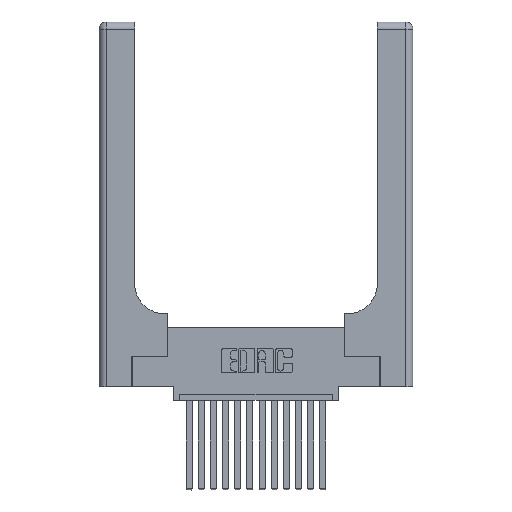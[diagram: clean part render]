
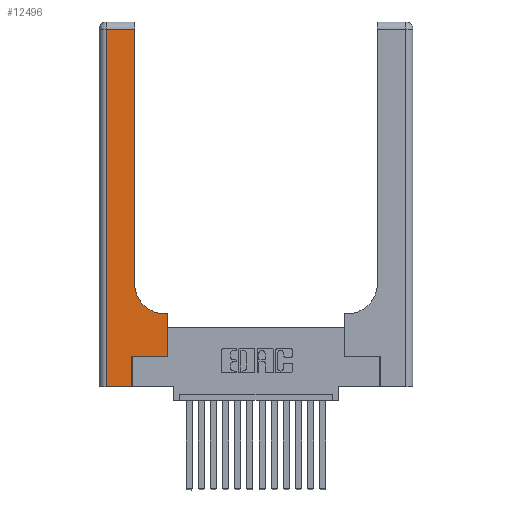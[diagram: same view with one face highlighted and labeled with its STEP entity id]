
A CAD part, top view. The second image highlights one B-rep face of the part: STEP entity #12496.
In plain terms, the highlighted planar face has unit normal (0, 0, 1).
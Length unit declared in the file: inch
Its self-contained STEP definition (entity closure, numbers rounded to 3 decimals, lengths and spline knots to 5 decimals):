
#476 = EDGE_CURVE ( 'NONE', #5047, #6004, #5724, .T. ) ;
#490 = CARTESIAN_POINT ( 'NONE',  ( 0.269, 0., 0.37 ) ) ;
#1063 = ORIENTED_EDGE ( 'NONE', *, *, #13172, .T. ) ;
#1244 = DIRECTION ( 'NONE',  ( 0., 1., 0. ) ) ;
#1622 = DIRECTION ( 'NONE',  ( -1., 0., 0. ) ) ;
#2347 = CARTESIAN_POINT ( 'NONE',  ( 0.269, 0.25, 0.37 ) ) ;
#2625 = EDGE_CURVE ( 'NONE', #14415, #11265, #12244, .T. ) ;
#2713 = CARTESIAN_POINT ( 'NONE',  ( 0.5585, 0.25, 0.37 ) ) ;
#2748 = DIRECTION ( 'NONE',  ( 1., 0., 0. ) ) ;
#2900 = ORIENTED_EDGE ( 'NONE', *, *, #7976, .T. ) ;
#3698 = DIRECTION ( 'NONE',  ( 0., 0., -1. ) ) ;
#3905 = VERTEX_POINT ( 'NONE', #13293 ) ;
#4234 = CARTESIAN_POINT ( 'NONE',  ( 0.2915, 0.6, 0.37 ) ) ;
#4484 = DIRECTION ( 'NONE',  ( 1., 0., 0. ) ) ;
#5047 = VERTEX_POINT ( 'NONE', #8200 ) ;
#5060 = LINE ( 'NONE', #4234, #17176 ) ;
#5097 = DIRECTION ( 'NONE',  ( 1., 0., 0. ) ) ;
#5101 = ORIENTED_EDGE ( 'NONE', *, *, #476, .T. ) ;
#5525 = CARTESIAN_POINT ( 'NONE',  ( 0.06, 3., 0.37 ) ) ;
#5642 = FACE_OUTER_BOUND ( 'NONE', #10318, .T. ) ;
#5724 = LINE ( 'NONE', #11470, #12752 ) ;
#6004 = VERTEX_POINT ( 'NONE', #490 ) ;
#6273 = EDGE_CURVE ( 'NONE', #8049, #10556, #16321, .T. ) ;
#7059 = VERTEX_POINT ( 'NONE', #11774 ) ;
#7067 = CARTESIAN_POINT ( 'NONE',  ( 0.269, 0.25, 0.37 ) ) ;
#7163 = CARTESIAN_POINT ( 'NONE',  ( 0.5585, 0.6, 0.37 ) ) ;
#7392 = LINE ( 'NONE', #2713, #18191 ) ;
#7620 = DIRECTION ( 'NONE',  ( -1., 0., 0. ) ) ;
#7970 = ORIENTED_EDGE ( 'NONE', *, *, #9755, .T. ) ;
#7974 = CARTESIAN_POINT ( 'NONE',  ( 0.5415, 0.85, 0.37 ) ) ;
#7976 = EDGE_CURVE ( 'NONE', #6004, #14415, #17235, .T. ) ;
#7995 = CARTESIAN_POINT ( 'NONE',  ( 0., 2.94, 0.37 ) ) ;
#8049 = VERTEX_POINT ( 'NONE', #11360 ) ;
#8055 = DIRECTION ( 'NONE',  ( -1., 0., 0. ) ) ;
#8200 = CARTESIAN_POINT ( 'NONE',  ( 0.06, 0., 0.37 ) ) ;
#8495 = ORIENTED_EDGE ( 'NONE', *, *, #13128, .T. ) ;
#8519 = VECTOR ( 'NONE', #2748, 39.37008 ) ;
#9462 = AXIS2_PLACEMENT_3D ( 'NONE', #7974, #3698, #5097 ) ;
#9755 = EDGE_CURVE ( 'NONE', #13922, #8049, #5060, .T. ) ;
#10318 = EDGE_LOOP ( 'NONE', ( #1063, #11542, #17519, #5101, #2900, #17037, #8495, #7970, #16555 ) ) ;
#10556 = VERTEX_POINT ( 'NONE', #16542 ) ;
#10917 = DIRECTION ( 'NONE',  ( 0., -1., 0. ) ) ;
#11120 = EDGE_CURVE ( 'NONE', #7059, #5047, #15314, .T. ) ;
#11265 = VERTEX_POINT ( 'NONE', #12883 ) ;
#11360 = CARTESIAN_POINT ( 'NONE',  ( 0.5415, 0.6, 0.37 ) ) ;
#11470 = CARTESIAN_POINT ( 'NONE',  ( 0., 0., 0.37 ) ) ;
#11542 = ORIENTED_EDGE ( 'NONE', *, *, #17731, .T. ) ;
#11727 = DIRECTION ( 'NONE',  ( 0., 0., -1. ) ) ;
#11774 = CARTESIAN_POINT ( 'NONE',  ( 0.06, 2.94, 0.37 ) ) ;
#11973 = CARTESIAN_POINT ( 'NONE',  ( 0., 3., 0.37 ) ) ;
#12244 = LINE ( 'NONE', #7067, #8519 ) ;
#12496 = ADVANCED_FACE ( 'NONE', ( #5642 ), #16056, .F. ) ;
#12752 = VECTOR ( 'NONE', #4484, 39.37008 ) ;
#12883 = CARTESIAN_POINT ( 'NONE',  ( 0.5585, 0.25, 0.37 ) ) ;
#13128 = EDGE_CURVE ( 'NONE', #11265, #13922, #7392, .T. ) ;
#13172 = EDGE_CURVE ( 'NONE', #10556, #3905, #17965, .T. ) ;
#13259 = CARTESIAN_POINT ( 'NONE',  ( 0.269, 0., 0.37 ) ) ;
#13293 = CARTESIAN_POINT ( 'NONE',  ( 0.2915, 2.94, 0.37 ) ) ;
#13842 = CARTESIAN_POINT ( 'NONE',  ( 0.2915, 3., 0.37 ) ) ;
#13902 = DIRECTION ( 'NONE',  ( 0., 1., 0. ) ) ;
#13922 = VERTEX_POINT ( 'NONE', #7163 ) ;
#14415 = VERTEX_POINT ( 'NONE', #2347 ) ;
#15314 = LINE ( 'NONE', #5525, #16684 ) ;
#15370 = AXIS2_PLACEMENT_3D ( 'NONE', #11973, #11727, #7620 ) ;
#15416 = VECTOR ( 'NONE', #8055, 39.37008 ) ;
#15877 = LINE ( 'NONE', #7995, #15416 ) ;
#16056 = PLANE ( 'NONE',  #15370 ) ;
#16321 = CIRCLE ( 'NONE', #9462, 0.25 ) ;
#16542 = CARTESIAN_POINT ( 'NONE',  ( 0.2915, 0.85, 0.37 ) ) ;
#16555 = ORIENTED_EDGE ( 'NONE', *, *, #6273, .T. ) ;
#16684 = VECTOR ( 'NONE', #10917, 39.37008 ) ;
#16796 = VECTOR ( 'NONE', #1244, 39.37008 ) ;
#17037 = ORIENTED_EDGE ( 'NONE', *, *, #2625, .T. ) ;
#17086 = VECTOR ( 'NONE', #13902, 39.37008 ) ;
#17176 = VECTOR ( 'NONE', #1622, 39.37008 ) ;
#17235 = LINE ( 'NONE', #13259, #16796 ) ;
#17519 = ORIENTED_EDGE ( 'NONE', *, *, #11120, .T. ) ;
#17731 = EDGE_CURVE ( 'NONE', #3905, #7059, #15877, .T. ) ;
#17965 = LINE ( 'NONE', #13842, #17086 ) ;
#18070 = DIRECTION ( 'NONE',  ( 0., 1., 0. ) ) ;
#18191 = VECTOR ( 'NONE', #18070, 39.37008 ) ;
